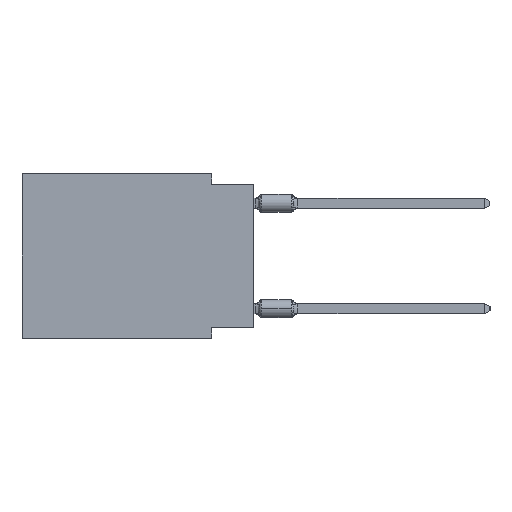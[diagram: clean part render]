
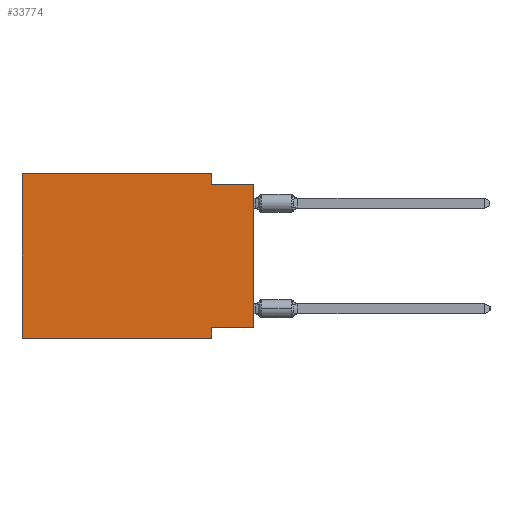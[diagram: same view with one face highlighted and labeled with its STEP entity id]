
A CAD part, left-side view. The second image highlights one B-rep face of the part: STEP entity #33774.
In plain terms, the highlighted planar face has unit normal (-1, 0, 0).
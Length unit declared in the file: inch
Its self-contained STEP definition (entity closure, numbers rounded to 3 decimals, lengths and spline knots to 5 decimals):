
#413 = CARTESIAN_POINT ( 'NONE',  ( 0., 0.1, -0.39 ) ) ;
#731 = LINE ( 'NONE', #19885, #11492 ) ;
#812 = CARTESIAN_POINT ( 'NONE',  ( 0., 0., -0.025 ) ) ;
#1570 = VERTEX_POINT ( 'NONE', #413 ) ;
#1576 = ORIENTED_EDGE ( 'NONE', *, *, #30542, .T. ) ;
#2413 = CARTESIAN_POINT ( 'NONE',  ( 0., 0.1, -0.365 ) ) ;
#2908 = ORIENTED_EDGE ( 'NONE', *, *, #8718, .F. ) ;
#2958 = VERTEX_POINT ( 'NONE', #812 ) ;
#3528 = DIRECTION ( 'NONE',  ( 1., 0., 0. ) ) ;
#5277 = LINE ( 'NONE', #53283, #60127 ) ;
#7466 = VERTEX_POINT ( 'NONE', #2413 ) ;
#8718 = EDGE_CURVE ( 'NONE', #29561, #55262, #53510, .T. ) ;
#9079 = ORIENTED_EDGE ( 'NONE', *, *, #43410, .F. ) ;
#10279 = DIRECTION ( 'NONE',  ( 0., -1., 0. ) ) ;
#11492 = VECTOR ( 'NONE', #39005, 39.37008 ) ;
#12007 = VERTEX_POINT ( 'NONE', #38985 ) ;
#12492 = CARTESIAN_POINT ( 'NONE',  ( 0., 0.55, 0. ) ) ;
#13126 = CARTESIAN_POINT ( 'NONE',  ( 0., 0.55, 0. ) ) ;
#14263 = DIRECTION ( 'NONE',  ( 0., 0., 1. ) ) ;
#14274 = ORIENTED_EDGE ( 'NONE', *, *, #22619, .F. ) ;
#15375 = DIRECTION ( 'NONE',  ( 0., 0., -1. ) ) ;
#19885 = CARTESIAN_POINT ( 'NONE',  ( 0., 0.55, 0. ) ) ;
#20236 = LINE ( 'NONE', #28397, #50429 ) ;
#22619 = EDGE_CURVE ( 'NONE', #51452, #2958, #59146, .T. ) ;
#22769 = CARTESIAN_POINT ( 'NONE',  ( 0., 0., -0.365 ) ) ;
#24480 = VECTOR ( 'NONE', #60068, 39.37008 ) ;
#26388 = EDGE_CURVE ( 'NONE', #12007, #7466, #36878, .T. ) ;
#26487 = CARTESIAN_POINT ( 'NONE',  ( 0., 0., -0.025 ) ) ;
#27071 = DIRECTION ( 'NONE',  ( 0., 0., -1. ) ) ;
#27381 = CARTESIAN_POINT ( 'NONE',  ( 0., 0.55, 0. ) ) ;
#28397 = CARTESIAN_POINT ( 'NONE',  ( 0., 0., 0. ) ) ;
#29147 = CARTESIAN_POINT ( 'NONE',  ( 0., 0.1, -0.39 ) ) ;
#29561 = VERTEX_POINT ( 'NONE', #61297 ) ;
#30370 = LINE ( 'NONE', #29147, #57858 ) ;
#30542 = EDGE_CURVE ( 'NONE', #29561, #1570, #5277, .T. ) ;
#31156 = FACE_OUTER_BOUND ( 'NONE', #55413, .T. ) ;
#32035 = ORIENTED_EDGE ( 'NONE', *, *, #42317, .F. ) ;
#33704 = ORIENTED_EDGE ( 'NONE', *, *, #26388, .F. ) ;
#33774 = ADVANCED_FACE ( 'NONE', ( #31156 ), #36784, .F. ) ;
#34172 = AXIS2_PLACEMENT_3D ( 'NONE', #27381, #3528, #27071 ) ;
#34513 = CARTESIAN_POINT ( 'NONE',  ( 0., 0.1, 0. ) ) ;
#35294 = EDGE_CURVE ( 'NONE', #12007, #2958, #20236, .T. ) ;
#36753 = CARTESIAN_POINT ( 'NONE',  ( 0., 0.1, 0. ) ) ;
#36784 = PLANE ( 'NONE',  #34172 ) ;
#36874 = VECTOR ( 'NONE', #15375, 39.37008 ) ;
#36878 = LINE ( 'NONE', #22769, #50856 ) ;
#36923 = EDGE_CURVE ( 'NONE', #55262, #44526, #731, .T. ) ;
#38985 = CARTESIAN_POINT ( 'NONE',  ( 0., 0., -0.365 ) ) ;
#39005 = DIRECTION ( 'NONE',  ( 0., -1., 0. ) ) ;
#41518 = CARTESIAN_POINT ( 'NONE',  ( 0., 0.1, -0.025 ) ) ;
#42060 = VECTOR ( 'NONE', #46673, 39.37008 ) ;
#42317 = EDGE_CURVE ( 'NONE', #7466, #1570, #30370, .T. ) ;
#43410 = EDGE_CURVE ( 'NONE', #44526, #51452, #58069, .T. ) ;
#43411 = ORIENTED_EDGE ( 'NONE', *, *, #35294, .T. ) ;
#44182 = DIRECTION ( 'NONE',  ( 0., 0., -1. ) ) ;
#44526 = VERTEX_POINT ( 'NONE', #36753 ) ;
#46673 = DIRECTION ( 'NONE',  ( 0., 0., 1. ) ) ;
#49022 = ORIENTED_EDGE ( 'NONE', *, *, #36923, .F. ) ;
#50429 = VECTOR ( 'NONE', #14263, 39.37008 ) ;
#50856 = VECTOR ( 'NONE', #61060, 39.37008 ) ;
#51452 = VERTEX_POINT ( 'NONE', #41518 ) ;
#53283 = CARTESIAN_POINT ( 'NONE',  ( 0., 0.55, -0.39 ) ) ;
#53510 = LINE ( 'NONE', #13126, #42060 ) ;
#55262 = VERTEX_POINT ( 'NONE', #12492 ) ;
#55413 = EDGE_LOOP ( 'NONE', ( #43411, #14274, #9079, #49022, #2908, #1576, #32035, #33704 ) ) ;
#57858 = VECTOR ( 'NONE', #44182, 39.37008 ) ;
#58069 = LINE ( 'NONE', #34513, #36874 ) ;
#59146 = LINE ( 'NONE', #26487, #24480 ) ;
#60068 = DIRECTION ( 'NONE',  ( 0., -1., 0. ) ) ;
#60127 = VECTOR ( 'NONE', #10279, 39.37008 ) ;
#61060 = DIRECTION ( 'NONE',  ( 0., 1., 0. ) ) ;
#61297 = CARTESIAN_POINT ( 'NONE',  ( 0., 0.55, -0.39 ) ) ;
